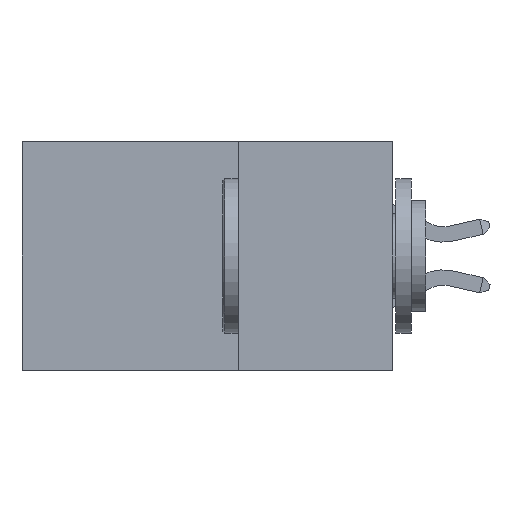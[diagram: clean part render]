
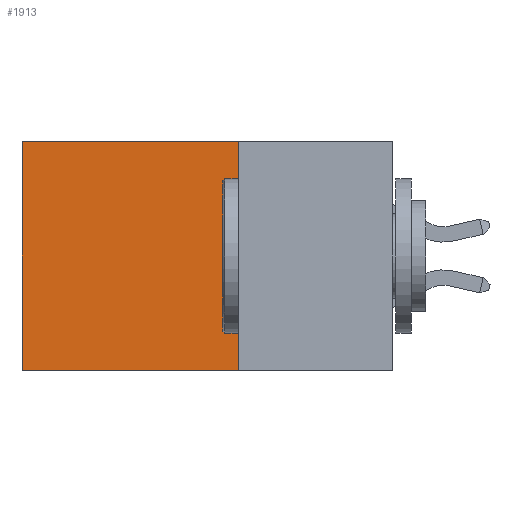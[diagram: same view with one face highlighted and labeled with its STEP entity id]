
A CAD part, left-side view. The second image highlights one B-rep face of the part: STEP entity #1913.
In plain terms, the highlighted planar face has unit normal (-1, 0, 0).
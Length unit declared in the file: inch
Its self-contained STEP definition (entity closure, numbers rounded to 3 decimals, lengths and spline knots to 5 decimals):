
#567 = DIRECTION ( 'NONE',  ( 0., 1., 0. ) ) ;
#749 = VECTOR ( 'NONE', #7907, 39.37008 ) ;
#946 = FACE_OUTER_BOUND ( 'NONE', #7775, .T. ) ;
#1075 = CARTESIAN_POINT ( 'NONE',  ( 0.2875, 0.25, -0.37 ) ) ;
#1740 = CARTESIAN_POINT ( 'NONE',  ( 0.2875, 0.6, 0. ) ) ;
#1913 = ADVANCED_FACE ( 'NONE', ( #946 ), #13533, .F. ) ;
#2570 = VECTOR ( 'NONE', #567, 39.37008 ) ;
#2828 = VERTEX_POINT ( 'NONE', #7458 ) ;
#3157 = DIRECTION ( 'NONE',  ( 1., 0., 0. ) ) ;
#3371 = VERTEX_POINT ( 'NONE', #10137 ) ;
#3656 = CARTESIAN_POINT ( 'NONE',  ( 0.2875, 0.25, -0.37 ) ) ;
#3855 = LINE ( 'NONE', #7421, #12505 ) ;
#6372 = EDGE_CURVE ( 'NONE', #2828, #10959, #10139, .T. ) ;
#7421 = CARTESIAN_POINT ( 'NONE',  ( 0.2875, 0.6, 0. ) ) ;
#7458 = CARTESIAN_POINT ( 'NONE',  ( 0.2875, 0.25, 0. ) ) ;
#7547 = CARTESIAN_POINT ( 'NONE',  ( 0.2875, 0.25, 0. ) ) ;
#7650 = CARTESIAN_POINT ( 'NONE',  ( 0.2875, 0.25, 0. ) ) ;
#7775 = EDGE_LOOP ( 'NONE', ( #11458, #12203, #14430, #9859 ) ) ;
#7907 = DIRECTION ( 'NONE',  ( 0., 1., 0. ) ) ;
#7955 = DIRECTION ( 'NONE',  ( 0., 0., -1. ) ) ;
#8895 = LINE ( 'NONE', #1075, #749 ) ;
#9859 = ORIENTED_EDGE ( 'NONE', *, *, #6372, .T. ) ;
#10137 = CARTESIAN_POINT ( 'NONE',  ( 0.2875, 0.6, -0.37 ) ) ;
#10139 = LINE ( 'NONE', #7547, #2570 ) ;
#10959 = VERTEX_POINT ( 'NONE', #1740 ) ;
#11076 = VECTOR ( 'NONE', #7955, 39.37008 ) ;
#11179 = DIRECTION ( 'NONE',  ( 0., 0., -1. ) ) ;
#11458 = ORIENTED_EDGE ( 'NONE', *, *, #13660, .T. ) ;
#11495 = VERTEX_POINT ( 'NONE', #3656 ) ;
#12203 = ORIENTED_EDGE ( 'NONE', *, *, #14405, .F. ) ;
#12282 = DIRECTION ( 'NONE',  ( 0., 0., -1. ) ) ;
#12323 = AXIS2_PLACEMENT_3D ( 'NONE', #7650, #3157, #12282 ) ;
#12505 = VECTOR ( 'NONE', #11179, 39.37008 ) ;
#12698 = LINE ( 'NONE', #14862, #11076 ) ;
#13365 = EDGE_CURVE ( 'NONE', #2828, #11495, #12698, .T. ) ;
#13533 = PLANE ( 'NONE',  #12323 ) ;
#13660 = EDGE_CURVE ( 'NONE', #10959, #3371, #3855, .T. ) ;
#14405 = EDGE_CURVE ( 'NONE', #11495, #3371, #8895, .T. ) ;
#14430 = ORIENTED_EDGE ( 'NONE', *, *, #13365, .F. ) ;
#14862 = CARTESIAN_POINT ( 'NONE',  ( 0.2875, 0.25, 0. ) ) ;
